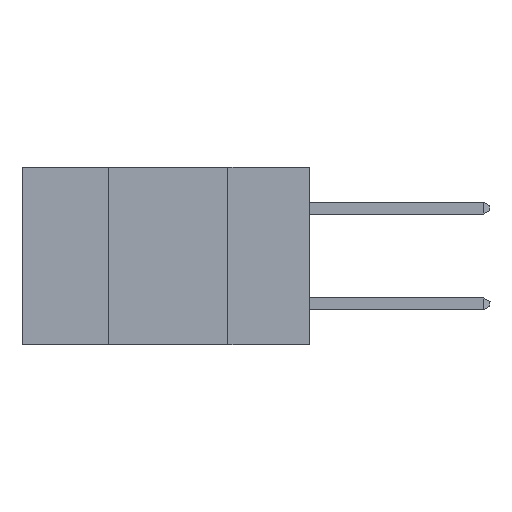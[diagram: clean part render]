
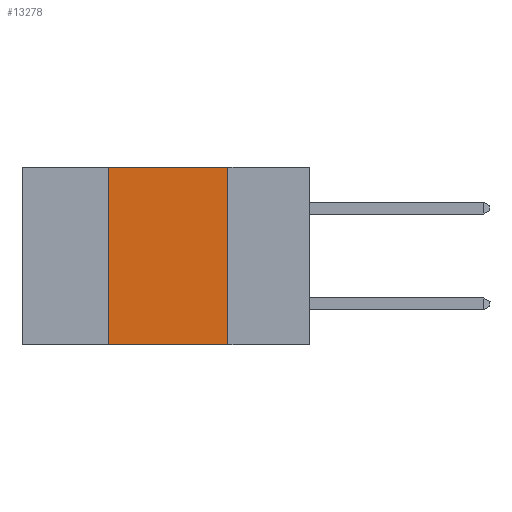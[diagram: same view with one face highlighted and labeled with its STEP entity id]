
A CAD part, left-side view. The second image highlights one B-rep face of the part: STEP entity #13278.
In plain terms, the highlighted planar face has unit normal (-1, 0, 0).
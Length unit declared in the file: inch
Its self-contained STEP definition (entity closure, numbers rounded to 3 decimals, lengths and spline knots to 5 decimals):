
#605 = VERTEX_POINT ( 'NONE', #10820 ) ;
#870 = VERTEX_POINT ( 'NONE', #2572 ) ;
#1175 = DIRECTION ( 'NONE',  ( 0., -1., 0. ) ) ;
#1698 = CARTESIAN_POINT ( 'NONE',  ( 0., 0.17, 0. ) ) ;
#2371 = DIRECTION ( 'NONE',  ( 0., 0., -1. ) ) ;
#2572 = CARTESIAN_POINT ( 'NONE',  ( 0., 0.42, -0.37 ) ) ;
#3171 = VECTOR ( 'NONE', #12006, 39.37008 ) ;
#3873 = VECTOR ( 'NONE', #10969, 39.37008 ) ;
#4710 = CARTESIAN_POINT ( 'NONE',  ( 0., 0.6, -0.37 ) ) ;
#5062 = PLANE ( 'NONE',  #11245 ) ;
#5085 = EDGE_CURVE ( 'NONE', #5716, #6721, #8269, .T. ) ;
#5558 = DIRECTION ( 'NONE',  ( 0., 0., -1. ) ) ;
#5716 = VERTEX_POINT ( 'NONE', #11175 ) ;
#6361 = EDGE_LOOP ( 'NONE', ( #14033, #9445, #14253, #9298 ) ) ;
#6721 = VERTEX_POINT ( 'NONE', #10302 ) ;
#6860 = EDGE_CURVE ( 'NONE', #6721, #605, #14744, .T. ) ;
#7665 = CARTESIAN_POINT ( 'NONE',  ( 0., 0.6, 0. ) ) ;
#8269 = LINE ( 'NONE', #14422, #3171 ) ;
#8453 = CARTESIAN_POINT ( 'NONE',  ( 0., 0.42, 0. ) ) ;
#9298 = ORIENTED_EDGE ( 'NONE', *, *, #10226, .T. ) ;
#9445 = ORIENTED_EDGE ( 'NONE', *, *, #5085, .F. ) ;
#10226 = EDGE_CURVE ( 'NONE', #870, #605, #11266, .T. ) ;
#10302 = CARTESIAN_POINT ( 'NONE',  ( 0., 0.17, 0. ) ) ;
#10820 = CARTESIAN_POINT ( 'NONE',  ( 0., 0.17, -0.37 ) ) ;
#10969 = DIRECTION ( 'NONE',  ( 0., 0., 1. ) ) ;
#11083 = EDGE_CURVE ( 'NONE', #870, #5716, #12444, .T. ) ;
#11140 = VECTOR ( 'NONE', #5558, 39.37008 ) ;
#11175 = CARTESIAN_POINT ( 'NONE',  ( 0., 0.42, 0. ) ) ;
#11245 = AXIS2_PLACEMENT_3D ( 'NONE', #7665, #13915, #2371 ) ;
#11266 = LINE ( 'NONE', #4710, #14906 ) ;
#12006 = DIRECTION ( 'NONE',  ( 0., -1., 0. ) ) ;
#12444 = LINE ( 'NONE', #8453, #3873 ) ;
#12755 = FACE_OUTER_BOUND ( 'NONE', #6361, .T. ) ;
#13278 = ADVANCED_FACE ( 'NONE', ( #12755 ), #5062, .F. ) ;
#13915 = DIRECTION ( 'NONE',  ( 1., 0., 0. ) ) ;
#14033 = ORIENTED_EDGE ( 'NONE', *, *, #6860, .F. ) ;
#14253 = ORIENTED_EDGE ( 'NONE', *, *, #11083, .F. ) ;
#14422 = CARTESIAN_POINT ( 'NONE',  ( 0., 0.6, 0. ) ) ;
#14744 = LINE ( 'NONE', #1698, #11140 ) ;
#14906 = VECTOR ( 'NONE', #1175, 39.37008 ) ;
